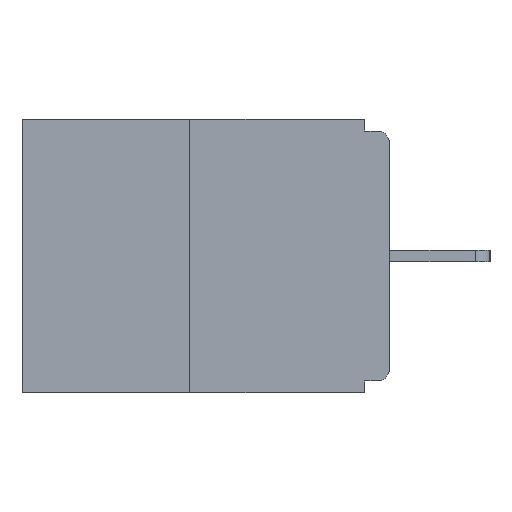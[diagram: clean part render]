
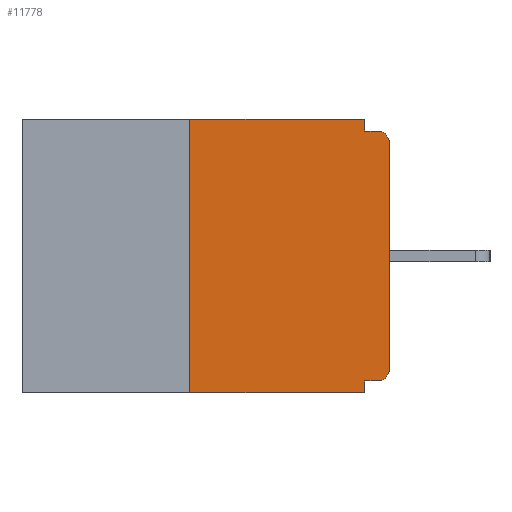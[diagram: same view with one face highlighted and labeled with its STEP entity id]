
A CAD part, left-side view. The second image highlights one B-rep face of the part: STEP entity #11778.
In plain terms, the highlighted planar face has unit normal (-1, 0, 0).
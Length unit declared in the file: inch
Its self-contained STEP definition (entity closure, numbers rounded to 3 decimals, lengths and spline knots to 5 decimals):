
#459 = CARTESIAN_POINT ( 'NONE',  ( 0., 0.015, -0.313 ) ) ;
#507 = AXIS2_PLACEMENT_3D ( 'NONE', #459, #14448, #1348 ) ;
#1348 = DIRECTION ( 'NONE',  ( 0., 0., -1. ) ) ;
#1450 = EDGE_CURVE ( 'NONE', #8579, #7705, #24653, .T. ) ;
#1669 = CARTESIAN_POINT ( 'NONE',  ( 0., 0., -0.03 ) ) ;
#2254 = VERTEX_POINT ( 'NONE', #12542 ) ;
#2778 = LINE ( 'NONE', #10715, #12152 ) ;
#2802 = DIRECTION ( 'NONE',  ( 0., -1., 0. ) ) ;
#2887 = VECTOR ( 'NONE', #3606, 39.37008 ) ;
#3606 = DIRECTION ( 'NONE',  ( 0., 1., 0. ) ) ;
#3906 = EDGE_LOOP ( 'NONE', ( #22458, #6500, #13574, #10359, #22578, #11713, #21204, #24179, #14429, #7499 ) ) ;
#3910 = LINE ( 'NONE', #4041, #24043 ) ;
#4041 = CARTESIAN_POINT ( 'NONE',  ( 0., 0., 0. ) ) ;
#4080 = LINE ( 'NONE', #12015, #12986 ) ;
#4218 = DIRECTION ( 'NONE',  ( 0., 0., -1. ) ) ;
#5262 = LINE ( 'NONE', #9159, #20918 ) ;
#5591 = EDGE_CURVE ( 'NONE', #23010, #6418, #7828, .T. ) ;
#5784 = CARTESIAN_POINT ( 'NONE',  ( 0., 0.015, -0.03 ) ) ;
#5876 = EDGE_CURVE ( 'NONE', #16704, #6418, #5262, .T. ) ;
#6418 = VERTEX_POINT ( 'NONE', #9254 ) ;
#6500 = ORIENTED_EDGE ( 'NONE', *, *, #9083, .F. ) ;
#6962 = EDGE_CURVE ( 'NONE', #7705, #16704, #4080, .T. ) ;
#7258 = DIRECTION ( 'NONE',  ( 0., 0., -1. ) ) ;
#7499 = ORIENTED_EDGE ( 'NONE', *, *, #6962, .F. ) ;
#7705 = VERTEX_POINT ( 'NONE', #14562 ) ;
#7711 = VERTEX_POINT ( 'NONE', #12172 ) ;
#7828 = CIRCLE ( 'NONE', #12016, 0.015 ) ;
#8302 = DIRECTION ( 'NONE',  ( 0., 0., -1. ) ) ;
#8368 = FACE_OUTER_BOUND ( 'NONE', #3906, .T. ) ;
#8579 = VERTEX_POINT ( 'NONE', #18285 ) ;
#9083 = EDGE_CURVE ( 'NONE', #7711, #8579, #2778, .T. ) ;
#9159 = CARTESIAN_POINT ( 'NONE',  ( 0., 0., -0.015 ) ) ;
#9254 = CARTESIAN_POINT ( 'NONE',  ( 0., 0.015, -0.015 ) ) ;
#9838 = EDGE_CURVE ( 'NONE', #2254, #21335, #19304, .T. ) ;
#10180 = DIRECTION ( 'NONE',  ( 0., 0., -1. ) ) ;
#10359 = ORIENTED_EDGE ( 'NONE', *, *, #10953, .F. ) ;
#10402 = CARTESIAN_POINT ( 'NONE',  ( 0., 0.031, -0.343 ) ) ;
#10684 = CARTESIAN_POINT ( 'NONE',  ( 0., 0.46, -0.343 ) ) ;
#10715 = CARTESIAN_POINT ( 'NONE',  ( 0., 0.25, 0. ) ) ;
#10953 = EDGE_CURVE ( 'NONE', #14330, #18459, #16189, .T. ) ;
#10998 = VECTOR ( 'NONE', #8302, 39.37008 ) ;
#11401 = AXIS2_PLACEMENT_3D ( 'NONE', #23844, #15990, #4218 ) ;
#11713 = ORIENTED_EDGE ( 'NONE', *, *, #9838, .T. ) ;
#11778 = ADVANCED_FACE ( 'NONE', ( #8368 ), #12440, .F. ) ;
#11838 = DIRECTION ( 'NONE',  ( 0., 0., 1. ) ) ;
#12015 = CARTESIAN_POINT ( 'NONE',  ( 0., 0.031, 0. ) ) ;
#12016 = AXIS2_PLACEMENT_3D ( 'NONE', #5784, #25798, #7258 ) ;
#12152 = VECTOR ( 'NONE', #14926, 39.37008 ) ;
#12172 = CARTESIAN_POINT ( 'NONE',  ( 0., 0.25, -0.343 ) ) ;
#12440 = PLANE ( 'NONE',  #11401 ) ;
#12542 = CARTESIAN_POINT ( 'NONE',  ( 0., 0.015, -0.328 ) ) ;
#12986 = VECTOR ( 'NONE', #10180, 39.37008 ) ;
#13574 = ORIENTED_EDGE ( 'NONE', *, *, #15018, .T. ) ;
#14219 = DIRECTION ( 'NONE',  ( 0., -1., 0. ) ) ;
#14330 = VERTEX_POINT ( 'NONE', #17648 ) ;
#14429 = ORIENTED_EDGE ( 'NONE', *, *, #5876, .F. ) ;
#14448 = DIRECTION ( 'NONE',  ( -1., 0., 0. ) ) ;
#14562 = CARTESIAN_POINT ( 'NONE',  ( 0., 0.031, 0. ) ) ;
#14926 = DIRECTION ( 'NONE',  ( 0., 0., 1. ) ) ;
#15018 = EDGE_CURVE ( 'NONE', #7711, #18459, #20249, .T. ) ;
#15700 = VECTOR ( 'NONE', #20734, 39.37008 ) ;
#15718 = CARTESIAN_POINT ( 'NONE',  ( 0., 0.031, -0.343 ) ) ;
#15748 = LINE ( 'NONE', #19795, #2887 ) ;
#15851 = CARTESIAN_POINT ( 'NONE',  ( 0., 0., -0.313 ) ) ;
#15990 = DIRECTION ( 'NONE',  ( 1., 0., 0. ) ) ;
#16189 = LINE ( 'NONE', #10402, #10998 ) ;
#16704 = VERTEX_POINT ( 'NONE', #20354 ) ;
#17648 = CARTESIAN_POINT ( 'NONE',  ( 0., 0.031, -0.328 ) ) ;
#18285 = CARTESIAN_POINT ( 'NONE',  ( 0., 0.25, 0. ) ) ;
#18459 = VERTEX_POINT ( 'NONE', #15718 ) ;
#19304 = CIRCLE ( 'NONE', #507, 0.015 ) ;
#19334 = EDGE_CURVE ( 'NONE', #21335, #23010, #3910, .T. ) ;
#19795 = CARTESIAN_POINT ( 'NONE',  ( 0., 0., -0.328 ) ) ;
#20249 = LINE ( 'NONE', #10684, #24780 ) ;
#20354 = CARTESIAN_POINT ( 'NONE',  ( 0., 0.031, -0.015 ) ) ;
#20734 = DIRECTION ( 'NONE',  ( 0., -1., 0. ) ) ;
#20918 = VECTOR ( 'NONE', #2802, 39.37008 ) ;
#21204 = ORIENTED_EDGE ( 'NONE', *, *, #19334, .T. ) ;
#21335 = VERTEX_POINT ( 'NONE', #15851 ) ;
#22285 = CARTESIAN_POINT ( 'NONE',  ( 0., 0.46, 0. ) ) ;
#22458 = ORIENTED_EDGE ( 'NONE', *, *, #1450, .F. ) ;
#22578 = ORIENTED_EDGE ( 'NONE', *, *, #23409, .F. ) ;
#23010 = VERTEX_POINT ( 'NONE', #1669 ) ;
#23409 = EDGE_CURVE ( 'NONE', #2254, #14330, #15748, .T. ) ;
#23844 = CARTESIAN_POINT ( 'NONE',  ( 0., 0.46, 0. ) ) ;
#24043 = VECTOR ( 'NONE', #11838, 39.37008 ) ;
#24179 = ORIENTED_EDGE ( 'NONE', *, *, #5591, .T. ) ;
#24653 = LINE ( 'NONE', #22285, #15700 ) ;
#24780 = VECTOR ( 'NONE', #14219, 39.37008 ) ;
#25798 = DIRECTION ( 'NONE',  ( -1., 0., 0. ) ) ;
